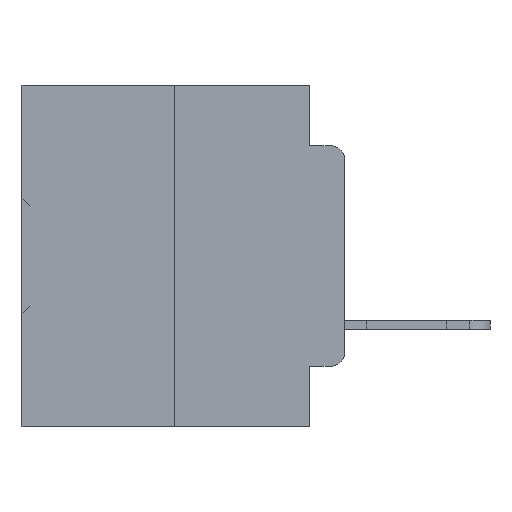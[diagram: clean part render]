
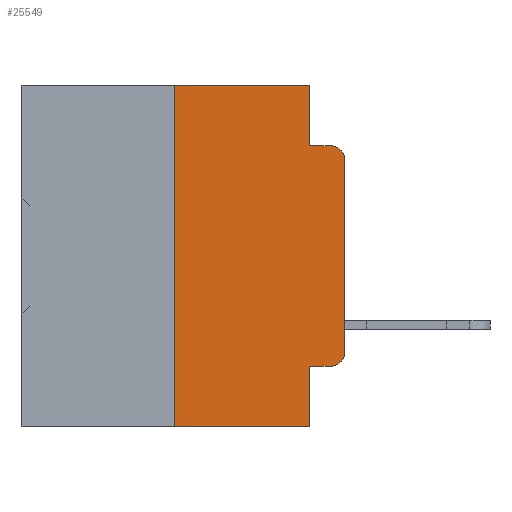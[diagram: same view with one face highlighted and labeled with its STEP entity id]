
A CAD part, left-side view. The second image highlights one B-rep face of the part: STEP entity #25549.
In plain terms, the highlighted planar face has unit normal (-1, 0, 0).
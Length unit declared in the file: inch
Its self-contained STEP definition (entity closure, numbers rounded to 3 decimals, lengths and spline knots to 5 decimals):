
#510 = CARTESIAN_POINT ( 'NONE',  ( 0., 0.051, 0. ) ) ;
#1737 = ORIENTED_EDGE ( 'NONE', *, *, #29064, .F. ) ;
#2321 = ORIENTED_EDGE ( 'NONE', *, *, #8308, .T. ) ;
#2803 = CARTESIAN_POINT ( 'NONE',  ( 0., 0.473, 0. ) ) ;
#3453 = EDGE_LOOP ( 'NONE', ( #15343, #2321, #25314, #1737, #13276, #6289, #15895, #30413, #17981, #9281 ) ) ;
#4192 = CARTESIAN_POINT ( 'NONE',  ( 0., 0.473, 0. ) ) ;
#4222 = DIRECTION ( 'NONE',  ( 0., 0., 1. ) ) ;
#4333 = LINE ( 'NONE', #32792, #13377 ) ;
#4589 = DIRECTION ( 'NONE',  ( -1., 0., 0. ) ) ;
#4869 = DIRECTION ( 'NONE',  ( -1., 0., 0. ) ) ;
#4933 = VERTEX_POINT ( 'NONE', #15714 ) ;
#5150 = CARTESIAN_POINT ( 'NONE',  ( 0., 0.25, -0.5 ) ) ;
#5496 = CARTESIAN_POINT ( 'NONE',  ( 0., 0.051, -0.4115 ) ) ;
#5632 = EDGE_CURVE ( 'NONE', #18661, #7887, #18127, .T. ) ;
#5663 = VECTOR ( 'NONE', #34274, 39.37008 ) ;
#6018 = VECTOR ( 'NONE', #20226, 39.37008 ) ;
#6260 = DIRECTION ( 'NONE',  ( 0., 0., -1. ) ) ;
#6289 = ORIENTED_EDGE ( 'NONE', *, *, #16902, .F. ) ;
#6647 = CARTESIAN_POINT ( 'NONE',  ( 0., 0.25, 0. ) ) ;
#6769 = VERTEX_POINT ( 'NONE', #11842 ) ;
#7518 = CARTESIAN_POINT ( 'NONE',  ( 0., 0.051, -0.4115 ) ) ;
#7887 = VERTEX_POINT ( 'NONE', #35173 ) ;
#8308 = EDGE_CURVE ( 'NONE', #6769, #7887, #14129, .T. ) ;
#8365 = EDGE_CURVE ( 'NONE', #18389, #36365, #20270, .T. ) ;
#9281 = ORIENTED_EDGE ( 'NONE', *, *, #27622, .T. ) ;
#9770 = EDGE_CURVE ( 'NONE', #10732, #4933, #16369, .T. ) ;
#10167 = LINE ( 'NONE', #28756, #38723 ) ;
#10732 = VERTEX_POINT ( 'NONE', #5496 ) ;
#11842 = CARTESIAN_POINT ( 'NONE',  ( 0., 0., -0.1085 ) ) ;
#13276 = ORIENTED_EDGE ( 'NONE', *, *, #8365, .F. ) ;
#13377 = VECTOR ( 'NONE', #32924, 39.37008 ) ;
#13396 = CIRCLE ( 'NONE', #19835, 0.02 ) ;
#13789 = LINE ( 'NONE', #510, #5663 ) ;
#13979 = CARTESIAN_POINT ( 'NONE',  ( 0., 0.473, -0.5 ) ) ;
#14129 = CIRCLE ( 'NONE', #19118, 0.02 ) ;
#14696 = CARTESIAN_POINT ( 'NONE',  ( 0., 0.051, 0. ) ) ;
#15073 = CARTESIAN_POINT ( 'NONE',  ( 0., 0., -0.3915 ) ) ;
#15339 = EDGE_CURVE ( 'NONE', #10732, #28562, #36420, .T. ) ;
#15343 = ORIENTED_EDGE ( 'NONE', *, *, #26391, .T. ) ;
#15362 = LINE ( 'NONE', #13979, #33897 ) ;
#15714 = CARTESIAN_POINT ( 'NONE',  ( 0., 0.051, -0.5 ) ) ;
#15895 = ORIENTED_EDGE ( 'NONE', *, *, #26950, .T. ) ;
#16369 = LINE ( 'NONE', #14696, #24392 ) ;
#16468 = AXIS2_PLACEMENT_3D ( 'NONE', #2803, #27342, #6260 ) ;
#16902 = EDGE_CURVE ( 'NONE', #37639, #18389, #4333, .T. ) ;
#17075 = DIRECTION ( 'NONE',  ( 0., 0., -1. ) ) ;
#17981 = ORIENTED_EDGE ( 'NONE', *, *, #15339, .T. ) ;
#18127 = LINE ( 'NONE', #30511, #27128 ) ;
#18389 = VERTEX_POINT ( 'NONE', #6647 ) ;
#18661 = VERTEX_POINT ( 'NONE', #26766 ) ;
#19118 = AXIS2_PLACEMENT_3D ( 'NONE', #31808, #4589, #28855 ) ;
#19835 = AXIS2_PLACEMENT_3D ( 'NONE', #26197, #4869, #17075 ) ;
#20226 = DIRECTION ( 'NONE',  ( 0., -1., 0. ) ) ;
#20270 = LINE ( 'NONE', #4192, #6018 ) ;
#21195 = VECTOR ( 'NONE', #23020, 39.37008 ) ;
#23020 = DIRECTION ( 'NONE',  ( 0., -1., 0. ) ) ;
#24392 = VECTOR ( 'NONE', #38646, 39.37008 ) ;
#25314 = ORIENTED_EDGE ( 'NONE', *, *, #5632, .F. ) ;
#25549 = ADVANCED_FACE ( 'NONE', ( #27403 ), #36164, .F. ) ;
#26197 = CARTESIAN_POINT ( 'NONE',  ( 0., 0.02, -0.3915 ) ) ;
#26391 = EDGE_CURVE ( 'NONE', #31811, #6769, #10167, .T. ) ;
#26766 = CARTESIAN_POINT ( 'NONE',  ( 0., 0.051, -0.0885 ) ) ;
#26950 = EDGE_CURVE ( 'NONE', #37639, #4933, #15362, .T. ) ;
#27128 = VECTOR ( 'NONE', #27569, 39.37008 ) ;
#27342 = DIRECTION ( 'NONE',  ( 1., 0., 0. ) ) ;
#27403 = FACE_OUTER_BOUND ( 'NONE', #3453, .T. ) ;
#27569 = DIRECTION ( 'NONE',  ( 0., -1., 0. ) ) ;
#27622 = EDGE_CURVE ( 'NONE', #28562, #31811, #13396, .T. ) ;
#28562 = VERTEX_POINT ( 'NONE', #34180 ) ;
#28756 = CARTESIAN_POINT ( 'NONE',  ( 0., 0., 0. ) ) ;
#28855 = DIRECTION ( 'NONE',  ( 0., 0., -1. ) ) ;
#29064 = EDGE_CURVE ( 'NONE', #36365, #18661, #13789, .T. ) ;
#30413 = ORIENTED_EDGE ( 'NONE', *, *, #9770, .F. ) ;
#30511 = CARTESIAN_POINT ( 'NONE',  ( 0., 0.051, -0.0885 ) ) ;
#31808 = CARTESIAN_POINT ( 'NONE',  ( 0., 0.02, -0.1085 ) ) ;
#31811 = VERTEX_POINT ( 'NONE', #15073 ) ;
#32221 = CARTESIAN_POINT ( 'NONE',  ( 0., 0.051, 0. ) ) ;
#32792 = CARTESIAN_POINT ( 'NONE',  ( 0., 0.25, 0. ) ) ;
#32924 = DIRECTION ( 'NONE',  ( 0., 0., 1. ) ) ;
#33897 = VECTOR ( 'NONE', #38032, 39.37008 ) ;
#34180 = CARTESIAN_POINT ( 'NONE',  ( 0., 0.02, -0.4115 ) ) ;
#34274 = DIRECTION ( 'NONE',  ( 0., 0., -1. ) ) ;
#35173 = CARTESIAN_POINT ( 'NONE',  ( 0., 0.02, -0.0885 ) ) ;
#36164 = PLANE ( 'NONE',  #16468 ) ;
#36365 = VERTEX_POINT ( 'NONE', #32221 ) ;
#36420 = LINE ( 'NONE', #7518, #21195 ) ;
#37639 = VERTEX_POINT ( 'NONE', #5150 ) ;
#38032 = DIRECTION ( 'NONE',  ( 0., -1., 0. ) ) ;
#38646 = DIRECTION ( 'NONE',  ( 0., 0., -1. ) ) ;
#38723 = VECTOR ( 'NONE', #4222, 39.37008 ) ;
